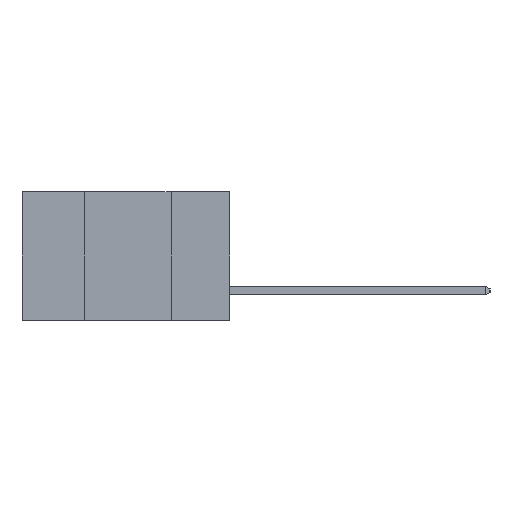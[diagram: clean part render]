
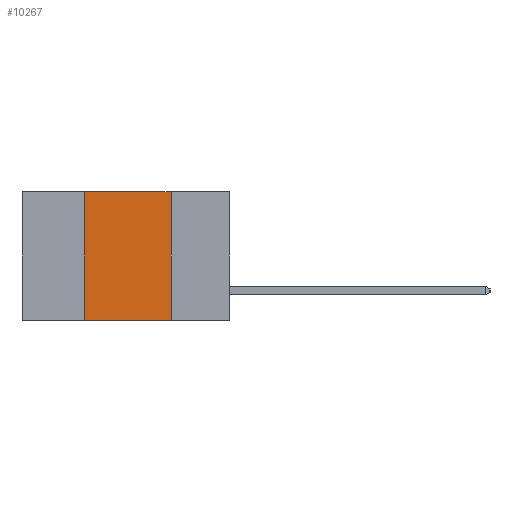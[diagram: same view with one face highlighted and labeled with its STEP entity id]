
A CAD part, left-side view. The second image highlights one B-rep face of the part: STEP entity #10267.
In plain terms, the highlighted planar face has unit normal (-1, 0, 0).
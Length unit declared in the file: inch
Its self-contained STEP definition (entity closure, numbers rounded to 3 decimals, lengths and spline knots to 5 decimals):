
#103 = EDGE_CURVE ( 'NONE', #1906, #499, #10626, .T. ) ;
#181 = DIRECTION ( 'NONE',  ( 0., -1., 0. ) ) ;
#499 = VERTEX_POINT ( 'NONE', #10329 ) ;
#816 = CARTESIAN_POINT ( 'NONE',  ( 0., 0.42, -0.37 ) ) ;
#901 = DIRECTION ( 'NONE',  ( 1., 0., 0. ) ) ;
#986 = ORIENTED_EDGE ( 'NONE', *, *, #14031, .T. ) ;
#1398 = CARTESIAN_POINT ( 'NONE',  ( 0., 0.42, 0. ) ) ;
#1906 = VERTEX_POINT ( 'NONE', #5783 ) ;
#3091 = VERTEX_POINT ( 'NONE', #816 ) ;
#3140 = ORIENTED_EDGE ( 'NONE', *, *, #103, .F. ) ;
#3465 = EDGE_LOOP ( 'NONE', ( #3140, #3637, #14877, #986 ) ) ;
#3637 = ORIENTED_EDGE ( 'NONE', *, *, #12788, .F. ) ;
#3756 = VERTEX_POINT ( 'NONE', #1398 ) ;
#3964 = CARTESIAN_POINT ( 'NONE',  ( 0., 0.42, 0. ) ) ;
#5783 = CARTESIAN_POINT ( 'NONE',  ( 0., 0.17, 0. ) ) ;
#6263 = LINE ( 'NONE', #11032, #8670 ) ;
#6363 = CARTESIAN_POINT ( 'NONE',  ( 0., 0.6, -0.37 ) ) ;
#6958 = PLANE ( 'NONE',  #8569 ) ;
#7511 = VECTOR ( 'NONE', #8594, 39.37008 ) ;
#7757 = CARTESIAN_POINT ( 'NONE',  ( 0., 0.17, 0. ) ) ;
#8535 = FACE_OUTER_BOUND ( 'NONE', #3465, .T. ) ;
#8569 = AXIS2_PLACEMENT_3D ( 'NONE', #15132, #901, #9314 ) ;
#8594 = DIRECTION ( 'NONE',  ( 0., 0., -1. ) ) ;
#8670 = VECTOR ( 'NONE', #181, 39.37008 ) ;
#8788 = LINE ( 'NONE', #6363, #11533 ) ;
#9314 = DIRECTION ( 'NONE',  ( 0., 0., -1. ) ) ;
#10267 = ADVANCED_FACE ( 'NONE', ( #8535 ), #6958, .F. ) ;
#10329 = CARTESIAN_POINT ( 'NONE',  ( 0., 0.17, -0.37 ) ) ;
#10626 = LINE ( 'NONE', #7757, #7511 ) ;
#11032 = CARTESIAN_POINT ( 'NONE',  ( 0., 0.6, 0. ) ) ;
#11533 = VECTOR ( 'NONE', #13417, 39.37008 ) ;
#11858 = LINE ( 'NONE', #3964, #15293 ) ;
#12239 = DIRECTION ( 'NONE',  ( 0., 0., 1. ) ) ;
#12788 = EDGE_CURVE ( 'NONE', #3756, #1906, #6263, .T. ) ;
#13417 = DIRECTION ( 'NONE',  ( 0., -1., 0. ) ) ;
#14031 = EDGE_CURVE ( 'NONE', #3091, #499, #8788, .T. ) ;
#14810 = EDGE_CURVE ( 'NONE', #3091, #3756, #11858, .T. ) ;
#14877 = ORIENTED_EDGE ( 'NONE', *, *, #14810, .F. ) ;
#15132 = CARTESIAN_POINT ( 'NONE',  ( 0., 0.6, 0. ) ) ;
#15293 = VECTOR ( 'NONE', #12239, 39.37008 ) ;
